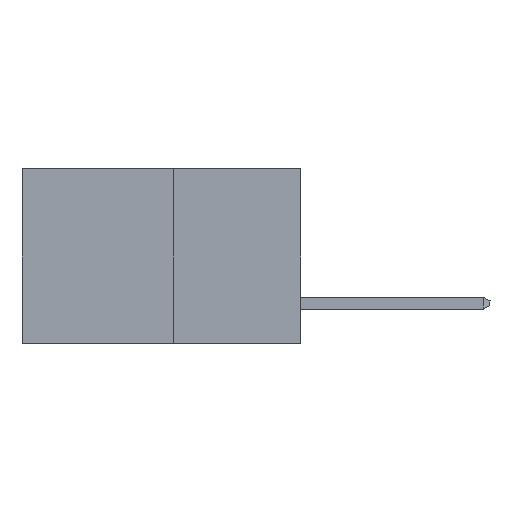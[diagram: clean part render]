
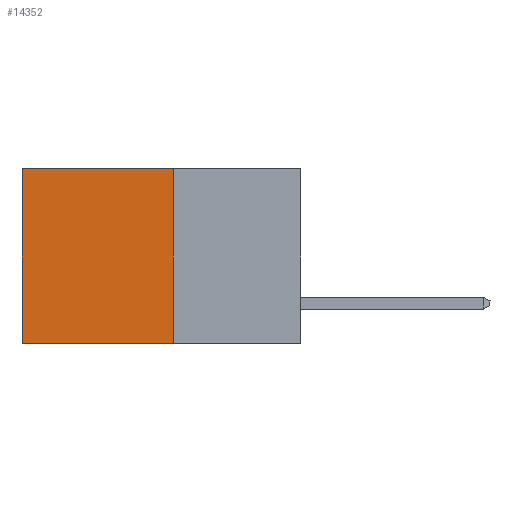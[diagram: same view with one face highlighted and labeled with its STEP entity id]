
A CAD part, left-side view. The second image highlights one B-rep face of the part: STEP entity #14352.
In plain terms, the highlighted planar face has unit normal (-1, 0, 0).
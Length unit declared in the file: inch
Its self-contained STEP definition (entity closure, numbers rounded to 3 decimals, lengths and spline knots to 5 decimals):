
#1242 = CARTESIAN_POINT ( 'NONE',  ( 0.277, 0.27, 0. ) ) ;
#2085 = VECTOR ( 'NONE', #15842, 39.37008 ) ;
#2731 = LINE ( 'NONE', #4580, #7070 ) ;
#2736 = PLANE ( 'NONE',  #15102 ) ;
#3248 = EDGE_CURVE ( 'NONE', #7140, #15296, #2731, .T. ) ;
#3416 = VECTOR ( 'NONE', #15783, 39.37008 ) ;
#3740 = CARTESIAN_POINT ( 'NONE',  ( 0.277, 0.59, -0.37 ) ) ;
#4064 = VERTEX_POINT ( 'NONE', #20450 ) ;
#4580 = CARTESIAN_POINT ( 'NONE',  ( 0.277, 0.27, -0.37 ) ) ;
#4587 = DIRECTION ( 'NONE',  ( 0., 0., -1. ) ) ;
#4924 = DIRECTION ( 'NONE',  ( 0., 0., -1. ) ) ;
#5015 = CARTESIAN_POINT ( 'NONE',  ( 0.277, 0.59, -0.37 ) ) ;
#5980 = FACE_OUTER_BOUND ( 'NONE', #13990, .T. ) ;
#7070 = VECTOR ( 'NONE', #4924, 39.37008 ) ;
#7140 = VERTEX_POINT ( 'NONE', #19620 ) ;
#7586 = EDGE_CURVE ( 'NONE', #7140, #4064, #22358, .T. ) ;
#7597 = LINE ( 'NONE', #5015, #2085 ) ;
#8916 = ORIENTED_EDGE ( 'NONE', *, *, #3248, .F. ) ;
#9186 = ORIENTED_EDGE ( 'NONE', *, *, #9232, .F. ) ;
#9232 = EDGE_CURVE ( 'NONE', #15296, #9815, #11975, .T. ) ;
#9583 = CARTESIAN_POINT ( 'NONE',  ( 0.277, 0.27, -0.37 ) ) ;
#9815 = VERTEX_POINT ( 'NONE', #3740 ) ;
#11975 = LINE ( 'NONE', #9583, #20659 ) ;
#13358 = ORIENTED_EDGE ( 'NONE', *, *, #20320, .T. ) ;
#13990 = EDGE_LOOP ( 'NONE', ( #13358, #9186, #8916, #21913 ) ) ;
#14352 = ADVANCED_FACE ( 'NONE', ( #5980 ), #2736, .F. ) ;
#15102 = AXIS2_PLACEMENT_3D ( 'NONE', #22308, #15447, #4587 ) ;
#15296 = VERTEX_POINT ( 'NONE', #16395 ) ;
#15447 = DIRECTION ( 'NONE',  ( 1., 0., 0. ) ) ;
#15783 = DIRECTION ( 'NONE',  ( 0., 1., 0. ) ) ;
#15842 = DIRECTION ( 'NONE',  ( 0., 0., -1. ) ) ;
#16395 = CARTESIAN_POINT ( 'NONE',  ( 0.277, 0.27, -0.37 ) ) ;
#19620 = CARTESIAN_POINT ( 'NONE',  ( 0.277, 0.27, 0. ) ) ;
#20073 = DIRECTION ( 'NONE',  ( 0., 1., 0. ) ) ;
#20320 = EDGE_CURVE ( 'NONE', #4064, #9815, #7597, .T. ) ;
#20450 = CARTESIAN_POINT ( 'NONE',  ( 0.277, 0.59, 0. ) ) ;
#20659 = VECTOR ( 'NONE', #20073, 39.37008 ) ;
#21913 = ORIENTED_EDGE ( 'NONE', *, *, #7586, .T. ) ;
#22308 = CARTESIAN_POINT ( 'NONE',  ( 0.277, 0.27, -0.37 ) ) ;
#22358 = LINE ( 'NONE', #1242, #3416 ) ;
